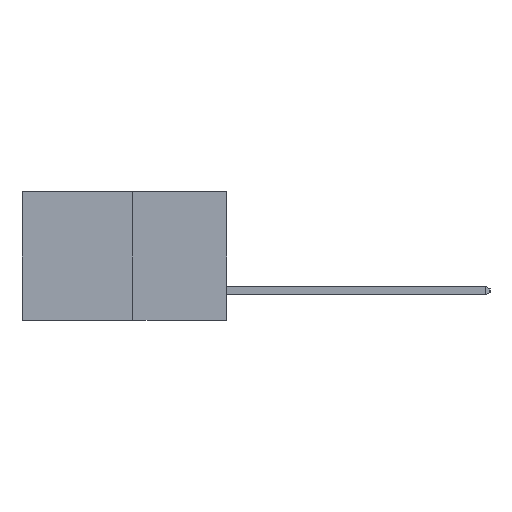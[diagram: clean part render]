
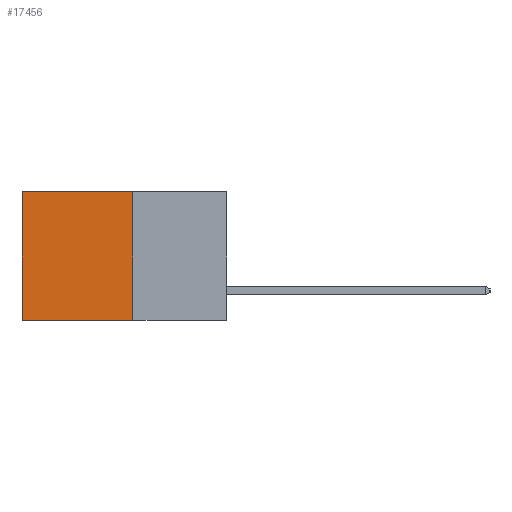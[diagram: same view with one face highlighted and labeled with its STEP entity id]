
A CAD part, left-side view. The second image highlights one B-rep face of the part: STEP entity #17456.
In plain terms, the highlighted planar face has unit normal (-1, 0, 0).
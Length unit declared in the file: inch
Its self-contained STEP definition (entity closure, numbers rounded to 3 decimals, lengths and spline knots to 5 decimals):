
#656 = DIRECTION ( 'NONE',  ( 0., 1., 0. ) ) ;
#723 = ORIENTED_EDGE ( 'NONE', *, *, #6923, .F. ) ;
#877 = VERTEX_POINT ( 'NONE', #10770 ) ;
#1339 = CARTESIAN_POINT ( 'NONE',  ( 0.277, 0.27, -0.37 ) ) ;
#2836 = DIRECTION ( 'NONE',  ( 0., 0., -1. ) ) ;
#3077 = VERTEX_POINT ( 'NONE', #16981 ) ;
#3403 = EDGE_CURVE ( 'NONE', #15753, #877, #6006, .T. ) ;
#4770 = LINE ( 'NONE', #9371, #16410 ) ;
#5600 = DIRECTION ( 'NONE',  ( 0., 0., -1. ) ) ;
#6006 = LINE ( 'NONE', #10129, #13448 ) ;
#6923 = EDGE_CURVE ( 'NONE', #3077, #877, #7566, .T. ) ;
#6973 = FACE_OUTER_BOUND ( 'NONE', #8024, .T. ) ;
#7099 = VECTOR ( 'NONE', #656, 39.37008 ) ;
#7566 = LINE ( 'NONE', #7995, #7099 ) ;
#7995 = CARTESIAN_POINT ( 'NONE',  ( 0.277, 0.27, -0.37 ) ) ;
#8004 = ORIENTED_EDGE ( 'NONE', *, *, #13779, .T. ) ;
#8024 = EDGE_LOOP ( 'NONE', ( #11833, #723, #11200, #8004 ) ) ;
#8349 = AXIS2_PLACEMENT_3D ( 'NONE', #1339, #11447, #2836 ) ;
#8706 = PLANE ( 'NONE',  #8349 ) ;
#9371 = CARTESIAN_POINT ( 'NONE',  ( 0.277, 0.27, 0. ) ) ;
#10129 = CARTESIAN_POINT ( 'NONE',  ( 0.277, 0.59, -0.37 ) ) ;
#10586 = CARTESIAN_POINT ( 'NONE',  ( 0.277, 0.27, 0. ) ) ;
#10770 = CARTESIAN_POINT ( 'NONE',  ( 0.277, 0.59, -0.37 ) ) ;
#11200 = ORIENTED_EDGE ( 'NONE', *, *, #14557, .F. ) ;
#11447 = DIRECTION ( 'NONE',  ( 1., 0., 0. ) ) ;
#11833 = ORIENTED_EDGE ( 'NONE', *, *, #3403, .T. ) ;
#12697 = VECTOR ( 'NONE', #5600, 39.37008 ) ;
#13448 = VECTOR ( 'NONE', #18197, 39.37008 ) ;
#13545 = CARTESIAN_POINT ( 'NONE',  ( 0.277, 0.59, 0. ) ) ;
#13779 = EDGE_CURVE ( 'NONE', #15631, #15753, #4770, .T. ) ;
#14015 = CARTESIAN_POINT ( 'NONE',  ( 0.277, 0.27, -0.37 ) ) ;
#14557 = EDGE_CURVE ( 'NONE', #15631, #3077, #17566, .T. ) ;
#15631 = VERTEX_POINT ( 'NONE', #10586 ) ;
#15753 = VERTEX_POINT ( 'NONE', #13545 ) ;
#16410 = VECTOR ( 'NONE', #17488, 39.37008 ) ;
#16981 = CARTESIAN_POINT ( 'NONE',  ( 0.277, 0.27, -0.37 ) ) ;
#17456 = ADVANCED_FACE ( 'NONE', ( #6973 ), #8706, .F. ) ;
#17488 = DIRECTION ( 'NONE',  ( 0., 1., 0. ) ) ;
#17566 = LINE ( 'NONE', #14015, #12697 ) ;
#18197 = DIRECTION ( 'NONE',  ( 0., 0., -1. ) ) ;
